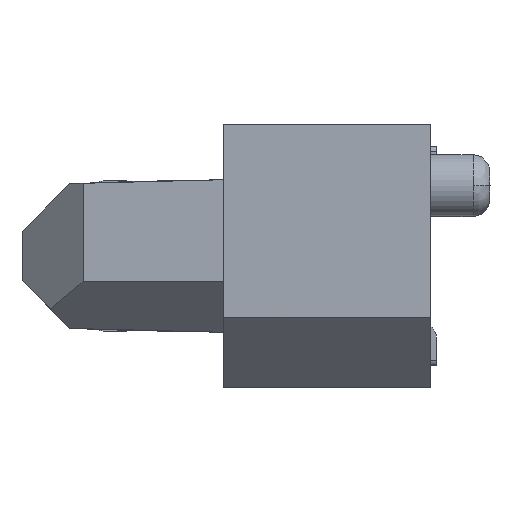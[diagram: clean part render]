
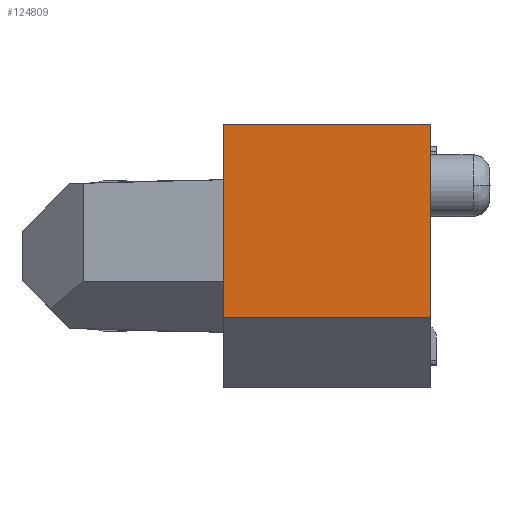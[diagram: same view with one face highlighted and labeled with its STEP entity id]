
A CAD part, left-side view. The second image highlights one B-rep face of the part: STEP entity #124809.
In plain terms, the highlighted planar face has unit normal (-1, 0, 0).
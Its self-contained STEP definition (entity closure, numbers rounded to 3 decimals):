
#520 = LINE ( 'NONE', #34247, #64991 ) ;
#837 = VERTEX_POINT ( 'NONE', #20738 ) ;
#2322 = VECTOR ( 'NONE', #34044, 1000. ) ;
#4518 = ORIENTED_EDGE ( 'NONE', *, *, #80381, .T. ) ;
#8890 = CARTESIAN_POINT ( 'NONE',  ( -23., 0., 0. ) ) ;
#12456 = LINE ( 'NONE', #143643, #129499 ) ;
#15006 = VERTEX_POINT ( 'NONE', #50373 ) ;
#20738 = CARTESIAN_POINT ( 'NONE',  ( -23., 0., -1.3 ) ) ;
#22535 = CARTESIAN_POINT ( 'NONE',  ( -23., -4.4, 2.8 ) ) ;
#24671 = VERTEX_POINT ( 'NONE', #22535 ) ;
#32734 = VECTOR ( 'NONE', #139261, 1000. ) ;
#34044 = DIRECTION ( 'NONE',  ( 0., -1., 0. ) ) ;
#34247 = CARTESIAN_POINT ( 'NONE',  ( -23., -2.2, -1.3 ) ) ;
#34845 = PLANE ( 'NONE',  #143326 ) ;
#38321 = EDGE_CURVE ( 'NONE', #15006, #837, #520, .T. ) ;
#44045 = LINE ( 'NONE', #8890, #32734 ) ;
#48407 = DIRECTION ( 'NONE',  ( 0., 0., 1. ) ) ;
#50373 = CARTESIAN_POINT ( 'NONE',  ( -23., -4.4, -1.3 ) ) ;
#58271 = CARTESIAN_POINT ( 'NONE',  ( -23., -2.2, 0.75 ) ) ;
#64991 = VECTOR ( 'NONE', #83333, 1000. ) ;
#72250 = LINE ( 'NONE', #119898, #2322 ) ;
#80381 = EDGE_CURVE ( 'NONE', #15006, #24671, #12456, .T. ) ;
#82417 = FACE_OUTER_BOUND ( 'NONE', #122580, .T. ) ;
#82883 = VERTEX_POINT ( 'NONE', #148043 ) ;
#83333 = DIRECTION ( 'NONE',  ( 0., 1., 0. ) ) ;
#104714 = ORIENTED_EDGE ( 'NONE', *, *, #38321, .F. ) ;
#114055 = ORIENTED_EDGE ( 'NONE', *, *, #151230, .F. ) ;
#119898 = CARTESIAN_POINT ( 'NONE',  ( -23., -2.2, 2.8 ) ) ;
#122580 = EDGE_LOOP ( 'NONE', ( #146315, #114055, #104714, #4518 ) ) ;
#124809 = ADVANCED_FACE ( 'NONE', ( #82417 ), #34845, .F. ) ;
#129499 = VECTOR ( 'NONE', #48407, 1000. ) ;
#139261 = DIRECTION ( 'NONE',  ( 0., 0., 1. ) ) ;
#139448 = DIRECTION ( 'NONE',  ( 0., 0., -1. ) ) ;
#143326 = AXIS2_PLACEMENT_3D ( 'NONE', #58271, #153465, #139448 ) ;
#143643 = CARTESIAN_POINT ( 'NONE',  ( -23., -4.4, 0.75 ) ) ;
#145009 = EDGE_CURVE ( 'NONE', #82883, #24671, #72250, .T. ) ;
#146315 = ORIENTED_EDGE ( 'NONE', *, *, #145009, .F. ) ;
#148043 = CARTESIAN_POINT ( 'NONE',  ( -23., 0., 2.8 ) ) ;
#151230 = EDGE_CURVE ( 'NONE', #837, #82883, #44045, .T. ) ;
#153465 = DIRECTION ( 'NONE',  ( 1., 0., 0. ) ) ;
